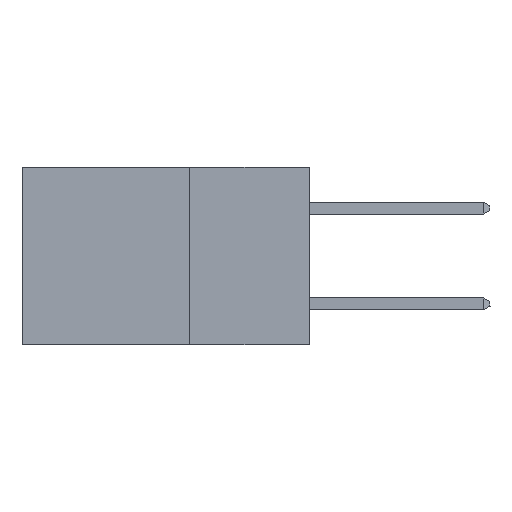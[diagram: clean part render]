
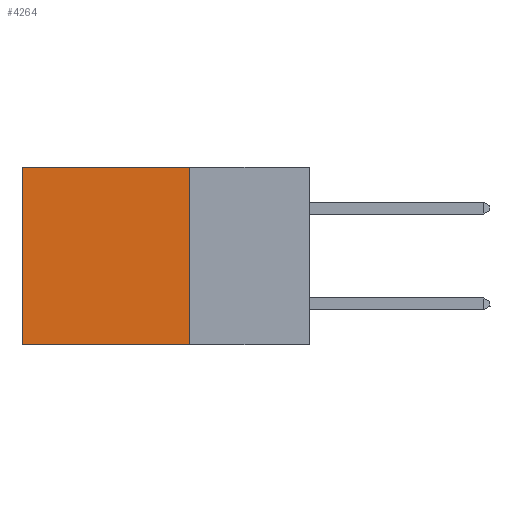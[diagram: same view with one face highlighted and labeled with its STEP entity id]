
A CAD part, left-side view. The second image highlights one B-rep face of the part: STEP entity #4264.
In plain terms, the highlighted planar face has unit normal (-1, 0, 0).
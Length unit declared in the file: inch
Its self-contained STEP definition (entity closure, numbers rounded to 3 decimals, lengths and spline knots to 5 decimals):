
#10 = CARTESIAN_POINT ( 'NONE',  ( 0.2875, 0.25, -0.37 ) ) ;
#1116 = EDGE_CURVE ( 'NONE', #12149, #22867, #16091, .T. ) ;
#1563 = VECTOR ( 'NONE', #16475, 39.37008 ) ;
#1767 = ORIENTED_EDGE ( 'NONE', *, *, #18168, .F. ) ;
#1836 = VERTEX_POINT ( 'NONE', #16418 ) ;
#2435 = DIRECTION ( 'NONE',  ( 0., 0., -1. ) ) ;
#3104 = LINE ( 'NONE', #17048, #13166 ) ;
#4264 = ADVANCED_FACE ( 'NONE', ( #22885 ), #14268, .F. ) ;
#5178 = AXIS2_PLACEMENT_3D ( 'NONE', #23374, #15929, #6583 ) ;
#6583 = DIRECTION ( 'NONE',  ( 0., 0., -1. ) ) ;
#7169 = VECTOR ( 'NONE', #13253, 39.37008 ) ;
#7744 = VERTEX_POINT ( 'NONE', #23020 ) ;
#12149 = VERTEX_POINT ( 'NONE', #22708 ) ;
#13060 = ORIENTED_EDGE ( 'NONE', *, *, #1116, .F. ) ;
#13166 = VECTOR ( 'NONE', #15277, 39.37008 ) ;
#13253 = DIRECTION ( 'NONE',  ( 0., 0., -1. ) ) ;
#13499 = CARTESIAN_POINT ( 'NONE',  ( 0.2875, 0.6, 0. ) ) ;
#13677 = LINE ( 'NONE', #21873, #1563 ) ;
#14268 = PLANE ( 'NONE',  #5178 ) ;
#15277 = DIRECTION ( 'NONE',  ( 0., 1., 0. ) ) ;
#15278 = LINE ( 'NONE', #13499, #19660 ) ;
#15929 = DIRECTION ( 'NONE',  ( 1., 0., 0. ) ) ;
#16091 = LINE ( 'NONE', #18739, #7169 ) ;
#16418 = CARTESIAN_POINT ( 'NONE',  ( 0.2875, 0.6, 0. ) ) ;
#16475 = DIRECTION ( 'NONE',  ( 0., 1., 0. ) ) ;
#17048 = CARTESIAN_POINT ( 'NONE',  ( 0.2875, 0.25, -0.37 ) ) ;
#18168 = EDGE_CURVE ( 'NONE', #22867, #7744, #3104, .T. ) ;
#18739 = CARTESIAN_POINT ( 'NONE',  ( 0.2875, 0.25, 0. ) ) ;
#19023 = EDGE_CURVE ( 'NONE', #12149, #1836, #13677, .T. ) ;
#19660 = VECTOR ( 'NONE', #2435, 39.37008 ) ;
#19857 = EDGE_LOOP ( 'NONE', ( #23245, #1767, #13060, #23203 ) ) ;
#21873 = CARTESIAN_POINT ( 'NONE',  ( 0.2875, 0.25, 0. ) ) ;
#21924 = EDGE_CURVE ( 'NONE', #1836, #7744, #15278, .T. ) ;
#22708 = CARTESIAN_POINT ( 'NONE',  ( 0.2875, 0.25, 0. ) ) ;
#22867 = VERTEX_POINT ( 'NONE', #10 ) ;
#22885 = FACE_OUTER_BOUND ( 'NONE', #19857, .T. ) ;
#23020 = CARTESIAN_POINT ( 'NONE',  ( 0.2875, 0.6, -0.37 ) ) ;
#23203 = ORIENTED_EDGE ( 'NONE', *, *, #19023, .T. ) ;
#23245 = ORIENTED_EDGE ( 'NONE', *, *, #21924, .T. ) ;
#23374 = CARTESIAN_POINT ( 'NONE',  ( 0.2875, 0.25, 0. ) ) ;
